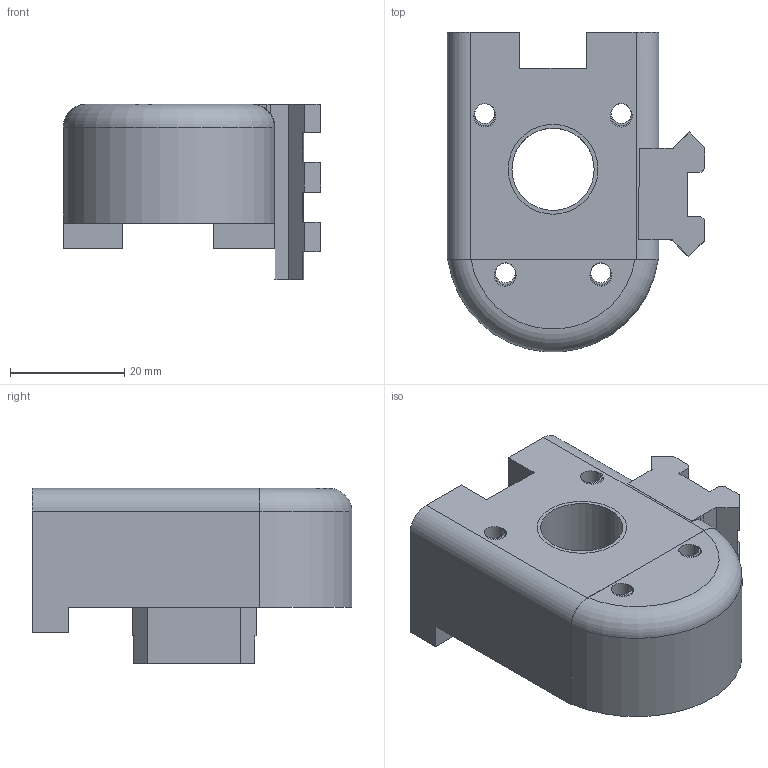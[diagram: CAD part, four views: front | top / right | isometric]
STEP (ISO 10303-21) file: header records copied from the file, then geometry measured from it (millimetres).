
FILE_DESCRIPTION(('FreeCAD Model'),'2;1');
FILE_NAME( 'ap9 barrel retainer.step' ,'2017-11-13T22:46:06',('Author'),(''), 'Open CASCADE STEP processor 6.8','FreeCAD','Unknown');
FILE_SCHEMA(('AUTOMOTIVE_DESIGN_CC2 { 1 2 10303 214 -1 1 5 4 }'));
Length unit declared in the file: millimetre
Products named in the file (1): Pocket002
Bounding box: 45.13 x 55.95 x 30.73 mm (x, y, z)
Volume: 37505.3 mm3; surface area: 10654.2 mm2
Topology: 1 solids, 2 shells, 132 faces, 394 edges, 270 vertices
Faces by surface type: plane 115, cylinder 16, torus 1
Full cylindrical faces by diameter (mm): 3.5 x4, 14.4 x1
Entity records: 10491 total; most frequent: CARTESIAN_POINT 2947, DIRECTION 1347, LINE 834, VECTOR 834, ORIENTED_EDGE 788, PCURVE 788, DEFINITIONAL_REPRESENTATION 788, EDGE_CURVE 394
